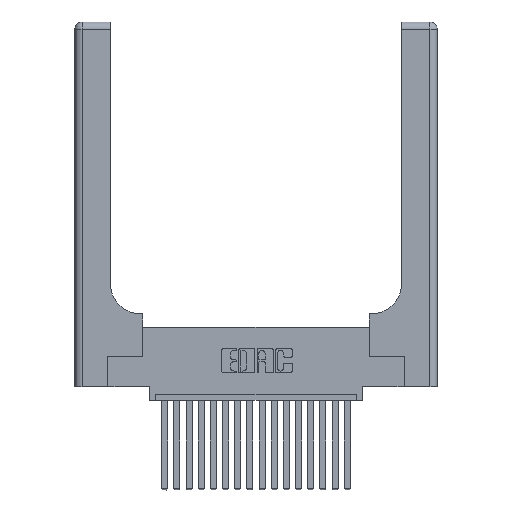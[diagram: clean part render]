
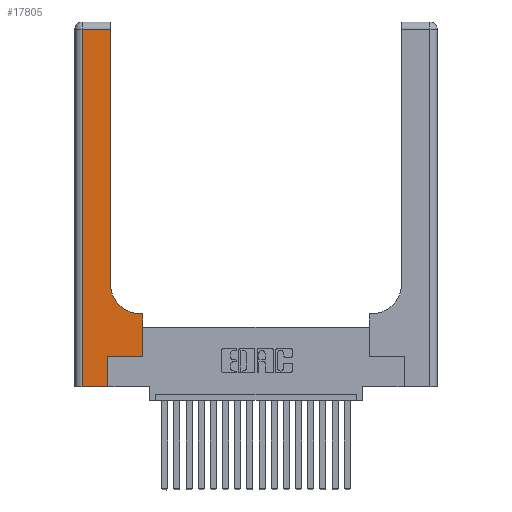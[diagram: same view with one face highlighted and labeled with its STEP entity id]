
A CAD part, top view. The second image highlights one B-rep face of the part: STEP entity #17805.
In plain terms, the highlighted planar face has unit normal (0, 0, 1).
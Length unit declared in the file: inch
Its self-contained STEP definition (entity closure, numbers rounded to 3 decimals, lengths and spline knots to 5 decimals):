
#386 = LINE ( 'NONE', #9744, #16866 ) ;
#388 = EDGE_CURVE ( 'NONE', #4854, #3900, #18440, .T. ) ;
#1090 = ORIENTED_EDGE ( 'NONE', *, *, #388, .T. ) ;
#1759 = EDGE_CURVE ( 'NONE', #18756, #19838, #5933, .T. ) ;
#2177 = DIRECTION ( 'NONE',  ( 0., 0., -1. ) ) ;
#2240 = DIRECTION ( 'NONE',  ( -1., 0., 0. ) ) ;
#3154 = ORIENTED_EDGE ( 'NONE', *, *, #12856, .T. ) ;
#3270 = VECTOR ( 'NONE', #16598, 39.37008 ) ;
#3540 = LINE ( 'NONE', #16522, #3270 ) ;
#3810 = LINE ( 'NONE', #5603, #14535 ) ;
#3900 = VERTEX_POINT ( 'NONE', #8904 ) ;
#4197 = CARTESIAN_POINT ( 'NONE',  ( 0.06, 3., 0.37 ) ) ;
#4322 = LINE ( 'NONE', #6298, #7791 ) ;
#4695 = ORIENTED_EDGE ( 'NONE', *, *, #15859, .T. ) ;
#4758 = CARTESIAN_POINT ( 'NONE',  ( 0.5415, 0.6, 0.37 ) ) ;
#4854 = VERTEX_POINT ( 'NONE', #11241 ) ;
#4905 = CARTESIAN_POINT ( 'NONE',  ( 0.269, 0.25, 0.37 ) ) ;
#5532 = ORIENTED_EDGE ( 'NONE', *, *, #1759, .T. ) ;
#5575 = ORIENTED_EDGE ( 'NONE', *, *, #14466, .T. ) ;
#5603 = CARTESIAN_POINT ( 'NONE',  ( 0.2915, 0.6, 0.37 ) ) ;
#5933 = LINE ( 'NONE', #7493, #18374 ) ;
#6298 = CARTESIAN_POINT ( 'NONE',  ( 0.5585, 0.25, 0.37 ) ) ;
#7252 = DIRECTION ( 'NONE',  ( 0., -1., 0. ) ) ;
#7493 = CARTESIAN_POINT ( 'NONE',  ( 0.2915, 3., 0.37 ) ) ;
#7791 = VECTOR ( 'NONE', #9562, 39.37008 ) ;
#8129 = CARTESIAN_POINT ( 'NONE',  ( 0.2915, 0.85, 0.37 ) ) ;
#8371 = ORIENTED_EDGE ( 'NONE', *, *, #15130, .T. ) ;
#8715 = EDGE_CURVE ( 'NONE', #19770, #18140, #15936, .T. ) ;
#8904 = CARTESIAN_POINT ( 'NONE',  ( 0.06, 0., 0.37 ) ) ;
#9562 = DIRECTION ( 'NONE',  ( 0., 1., 0. ) ) ;
#9744 = CARTESIAN_POINT ( 'NONE',  ( 0., 0., 0.37 ) ) ;
#10543 = VERTEX_POINT ( 'NONE', #12921 ) ;
#10752 = DIRECTION ( 'NONE',  ( 1., 0., 0. ) ) ;
#11241 = CARTESIAN_POINT ( 'NONE',  ( 0.06, 2.94, 0.37 ) ) ;
#11967 = CARTESIAN_POINT ( 'NONE',  ( 0.269, 0., 0.37 ) ) ;
#12007 = DIRECTION ( 'NONE',  ( -1., 0., 0. ) ) ;
#12169 = AXIS2_PLACEMENT_3D ( 'NONE', #17594, #16143, #19349 ) ;
#12322 = DIRECTION ( 'NONE',  ( 0., 1., 0. ) ) ;
#12574 = CIRCLE ( 'NONE', #12169, 0.25 ) ;
#12856 = EDGE_CURVE ( 'NONE', #3900, #19382, #386, .T. ) ;
#12921 = CARTESIAN_POINT ( 'NONE',  ( 0.5585, 0.6, 0.37 ) ) ;
#13265 = AXIS2_PLACEMENT_3D ( 'NONE', #16558, #2177, #18000 ) ;
#13474 = VECTOR ( 'NONE', #7252, 39.37008 ) ;
#13982 = ORIENTED_EDGE ( 'NONE', *, *, #15434, .T. ) ;
#14386 = CARTESIAN_POINT ( 'NONE',  ( 0.5585, 0.25, 0.37 ) ) ;
#14411 = CARTESIAN_POINT ( 'NONE',  ( 0.2915, 2.94, 0.37 ) ) ;
#14448 = VECTOR ( 'NONE', #10752, 39.37008 ) ;
#14466 = EDGE_CURVE ( 'NONE', #20318, #18756, #12574, .T. ) ;
#14535 = VECTOR ( 'NONE', #12007, 39.37008 ) ;
#14697 = VECTOR ( 'NONE', #2240, 39.37008 ) ;
#14962 = PLANE ( 'NONE',  #13265 ) ;
#15130 = EDGE_CURVE ( 'NONE', #18140, #10543, #4322, .T. ) ;
#15434 = EDGE_CURVE ( 'NONE', #10543, #20318, #3810, .T. ) ;
#15859 = EDGE_CURVE ( 'NONE', #19382, #19770, #3540, .T. ) ;
#15936 = LINE ( 'NONE', #20576, #14448 ) ;
#15978 = LINE ( 'NONE', #16809, #14697 ) ;
#16143 = DIRECTION ( 'NONE',  ( 0., 0., -1. ) ) ;
#16408 = ORIENTED_EDGE ( 'NONE', *, *, #16530, .T. ) ;
#16522 = CARTESIAN_POINT ( 'NONE',  ( 0.269, 0., 0.37 ) ) ;
#16530 = EDGE_CURVE ( 'NONE', #19838, #4854, #15978, .T. ) ;
#16558 = CARTESIAN_POINT ( 'NONE',  ( 0., 3., 0.37 ) ) ;
#16598 = DIRECTION ( 'NONE',  ( 0., 1., 0. ) ) ;
#16809 = CARTESIAN_POINT ( 'NONE',  ( 0., 2.94, 0.37 ) ) ;
#16866 = VECTOR ( 'NONE', #19170, 39.37008 ) ;
#16871 = EDGE_LOOP ( 'NONE', ( #5532, #16408, #1090, #3154, #4695, #18992, #8371, #13982, #5575 ) ) ;
#17594 = CARTESIAN_POINT ( 'NONE',  ( 0.5415, 0.85, 0.37 ) ) ;
#17805 = ADVANCED_FACE ( 'NONE', ( #19674 ), #14962, .F. ) ;
#18000 = DIRECTION ( 'NONE',  ( -1., 0., 0. ) ) ;
#18140 = VERTEX_POINT ( 'NONE', #14386 ) ;
#18374 = VECTOR ( 'NONE', #12322, 39.37008 ) ;
#18440 = LINE ( 'NONE', #4197, #13474 ) ;
#18756 = VERTEX_POINT ( 'NONE', #8129 ) ;
#18992 = ORIENTED_EDGE ( 'NONE', *, *, #8715, .T. ) ;
#19170 = DIRECTION ( 'NONE',  ( 1., 0., 0. ) ) ;
#19349 = DIRECTION ( 'NONE',  ( 1., 0., 0. ) ) ;
#19382 = VERTEX_POINT ( 'NONE', #11967 ) ;
#19674 = FACE_OUTER_BOUND ( 'NONE', #16871, .T. ) ;
#19770 = VERTEX_POINT ( 'NONE', #4905 ) ;
#19838 = VERTEX_POINT ( 'NONE', #14411 ) ;
#20318 = VERTEX_POINT ( 'NONE', #4758 ) ;
#20576 = CARTESIAN_POINT ( 'NONE',  ( 0.269, 0.25, 0.37 ) ) ;
